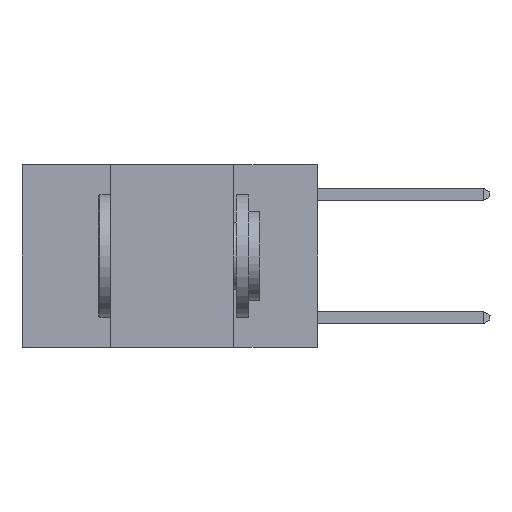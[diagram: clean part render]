
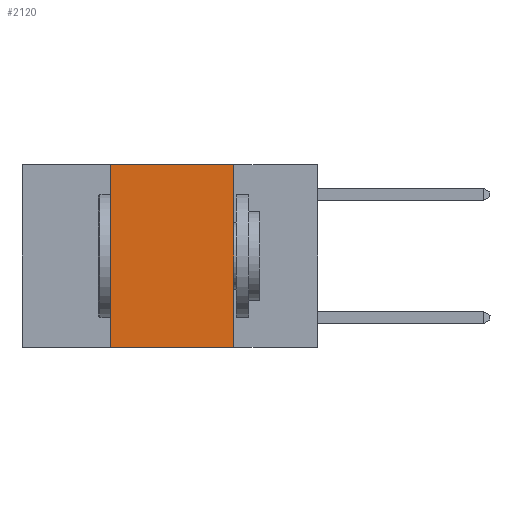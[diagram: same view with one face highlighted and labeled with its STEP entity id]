
A CAD part, left-side view. The second image highlights one B-rep face of the part: STEP entity #2120.
In plain terms, the highlighted planar face has unit normal (-1, 0, 0).
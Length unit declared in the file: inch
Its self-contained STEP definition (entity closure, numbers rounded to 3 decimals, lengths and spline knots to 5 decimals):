
#13 = LINE ( 'NONE', #7109, #8171 ) ;
#31 = VERTEX_POINT ( 'NONE', #1079 ) ;
#1077 = ORIENTED_EDGE ( 'NONE', *, *, #18351, .F. ) ;
#1079 = CARTESIAN_POINT ( 'NONE',  ( 0., 0.17, 0. ) ) ;
#1160 = ORIENTED_EDGE ( 'NONE', *, *, #7396, .F. ) ;
#1468 = ORIENTED_EDGE ( 'NONE', *, *, #10111, .F. ) ;
#1664 = ORIENTED_EDGE ( 'NONE', *, *, #7288, .T. ) ;
#1836 = CARTESIAN_POINT ( 'NONE',  ( 0., 0.6, 0. ) ) ;
#2120 = ADVANCED_FACE ( 'NONE', ( #18522 ), #15288, .F. ) ;
#2968 = CARTESIAN_POINT ( 'NONE',  ( 0., 0.42, -0.37 ) ) ;
#4311 = EDGE_LOOP ( 'NONE', ( #1077, #1160, #1468, #1664 ) ) ;
#7109 = CARTESIAN_POINT ( 'NONE',  ( 0., 0.6, -0.37 ) ) ;
#7288 = EDGE_CURVE ( 'NONE', #16320, #16772, #13, .T. ) ;
#7396 = EDGE_CURVE ( 'NONE', #13509, #31, #17712, .T. ) ;
#7417 = LINE ( 'NONE', #9050, #14775 ) ;
#7922 = DIRECTION ( 'NONE',  ( 0., 0., -1. ) ) ;
#8171 = VECTOR ( 'NONE', #17537, 39.37008 ) ;
#8193 = CARTESIAN_POINT ( 'NONE',  ( 0., 0.17, 0. ) ) ;
#9012 = VECTOR ( 'NONE', #9676, 39.37008 ) ;
#9050 = CARTESIAN_POINT ( 'NONE',  ( 0., 0.42, 0. ) ) ;
#9113 = DIRECTION ( 'NONE',  ( 0., 0., 1. ) ) ;
#9676 = DIRECTION ( 'NONE',  ( 0., 0., -1. ) ) ;
#10111 = EDGE_CURVE ( 'NONE', #16320, #13509, #7417, .T. ) ;
#10564 = AXIS2_PLACEMENT_3D ( 'NONE', #1836, #16831, #7922 ) ;
#11355 = CARTESIAN_POINT ( 'NONE',  ( 0., 0.17, -0.37 ) ) ;
#11735 = CARTESIAN_POINT ( 'NONE',  ( 0., 0.6, 0. ) ) ;
#13223 = DIRECTION ( 'NONE',  ( 0., -1., 0. ) ) ;
#13509 = VERTEX_POINT ( 'NONE', #16602 ) ;
#13732 = VECTOR ( 'NONE', #13223, 39.37008 ) ;
#14775 = VECTOR ( 'NONE', #9113, 39.37008 ) ;
#15288 = PLANE ( 'NONE',  #10564 ) ;
#16320 = VERTEX_POINT ( 'NONE', #2968 ) ;
#16481 = LINE ( 'NONE', #8193, #9012 ) ;
#16602 = CARTESIAN_POINT ( 'NONE',  ( 0., 0.42, 0. ) ) ;
#16772 = VERTEX_POINT ( 'NONE', #11355 ) ;
#16831 = DIRECTION ( 'NONE',  ( 1., 0., 0. ) ) ;
#17537 = DIRECTION ( 'NONE',  ( 0., -1., 0. ) ) ;
#17712 = LINE ( 'NONE', #11735, #13732 ) ;
#18351 = EDGE_CURVE ( 'NONE', #31, #16772, #16481, .T. ) ;
#18522 = FACE_OUTER_BOUND ( 'NONE', #4311, .T. ) ;
